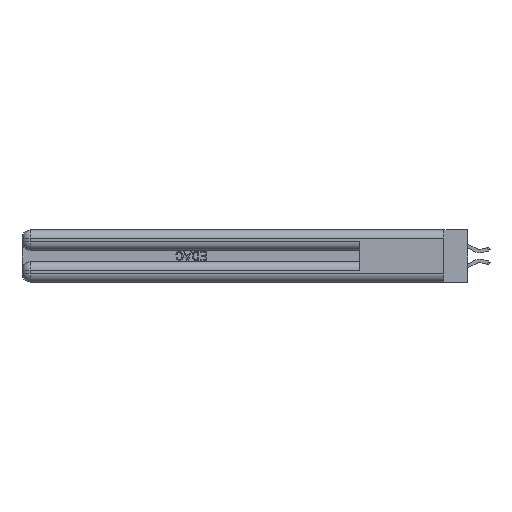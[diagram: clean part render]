
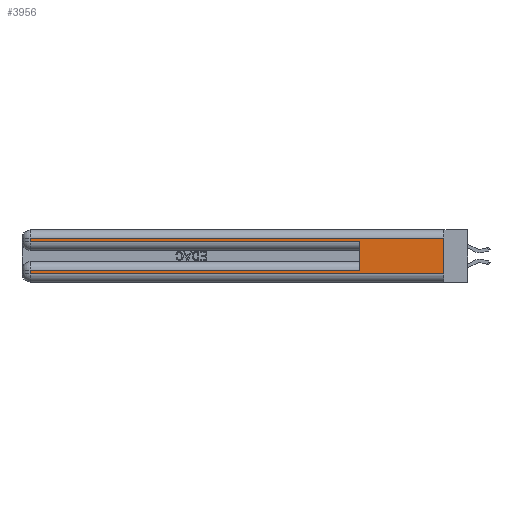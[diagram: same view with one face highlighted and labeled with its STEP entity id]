
A CAD part, left-side view. The second image highlights one B-rep face of the part: STEP entity #3956.
In plain terms, the highlighted planar face has unit normal (-1, 0, 0).
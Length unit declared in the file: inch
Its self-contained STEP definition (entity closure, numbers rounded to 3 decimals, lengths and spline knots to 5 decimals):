
#677 = DIRECTION ( 'NONE',  ( 0., 0., -1. ) ) ;
#1362 = ORIENTED_EDGE ( 'NONE', *, *, #16443, .T. ) ;
#1420 = LINE ( 'NONE', #37237, #9143 ) ;
#2358 = VERTEX_POINT ( 'NONE', #41826 ) ;
#2740 = VECTOR ( 'NONE', #677, 39.37008 ) ;
#3454 = CARTESIAN_POINT ( 'NONE',  ( 0., 0.6, 0.085 ) ) ;
#3956 = ADVANCED_FACE ( 'NONE', ( #18546 ), #12737, .F. ) ;
#4014 = CARTESIAN_POINT ( 'NONE',  ( 0., 2.94, 0.285 ) ) ;
#5277 = EDGE_CURVE ( 'NONE', #16732, #7262, #12969, .T. ) ;
#5862 = ORIENTED_EDGE ( 'NONE', *, *, #5277, .T. ) ;
#5980 = EDGE_CURVE ( 'NONE', #40839, #16732, #20058, .T. ) ;
#6211 = ORIENTED_EDGE ( 'NONE', *, *, #12853, .F. ) ;
#6799 = DIRECTION ( 'NONE',  ( 0., 0., 1. ) ) ;
#7092 = CARTESIAN_POINT ( 'NONE',  ( 0., 2.94, 0.37 ) ) ;
#7262 = VERTEX_POINT ( 'NONE', #27095 ) ;
#8301 = DIRECTION ( 'NONE',  ( 0., -1., 0. ) ) ;
#8622 = DIRECTION ( 'NONE',  ( 0., -1., 0. ) ) ;
#9143 = VECTOR ( 'NONE', #20192, 39.37008 ) ;
#9581 = LINE ( 'NONE', #7092, #37183 ) ;
#10175 = DIRECTION ( 'NONE',  ( 1., 0., 0. ) ) ;
#11609 = EDGE_CURVE ( 'NONE', #2358, #24197, #9581, .T. ) ;
#12737 = PLANE ( 'NONE',  #31847 ) ;
#12807 = ORIENTED_EDGE ( 'NONE', *, *, #5980, .T. ) ;
#12853 = EDGE_CURVE ( 'NONE', #19474, #7262, #25748, .T. ) ;
#12969 = LINE ( 'NONE', #24719, #32415 ) ;
#13239 = CARTESIAN_POINT ( 'NONE',  ( 0., 0., 0.37 ) ) ;
#13685 = CARTESIAN_POINT ( 'NONE',  ( 0., 2.94, 0.37 ) ) ;
#15417 = CARTESIAN_POINT ( 'NONE',  ( 0., 0., 0.37 ) ) ;
#15779 = ORIENTED_EDGE ( 'NONE', *, *, #11609, .T. ) ;
#16417 = CARTESIAN_POINT ( 'NONE',  ( 0., 0.6, 0.145 ) ) ;
#16443 = EDGE_CURVE ( 'NONE', #19474, #2358, #1420, .T. ) ;
#16732 = VERTEX_POINT ( 'NONE', #38180 ) ;
#18546 = FACE_OUTER_BOUND ( 'NONE', #22154, .T. ) ;
#19016 = ORIENTED_EDGE ( 'NONE', *, *, #34197, .T. ) ;
#19474 = VERTEX_POINT ( 'NONE', #27187 ) ;
#20058 = LINE ( 'NONE', #13685, #2740 ) ;
#20192 = DIRECTION ( 'NONE',  ( 0., 1., 0. ) ) ;
#20369 = CARTESIAN_POINT ( 'NONE',  ( 0., 0., 0.285 ) ) ;
#21607 = CARTESIAN_POINT ( 'NONE',  ( 0., 0., 0.085 ) ) ;
#22091 = LINE ( 'NONE', #16417, #39507 ) ;
#22154 = EDGE_LOOP ( 'NONE', ( #6211, #1362, #15779, #26830, #25198, #19016, #12807, #5862 ) ) ;
#23010 = DIRECTION ( 'NONE',  ( 0., 0., -1. ) ) ;
#24197 = VERTEX_POINT ( 'NONE', #4014 ) ;
#24719 = CARTESIAN_POINT ( 'NONE',  ( 0., 0., 0.06 ) ) ;
#24975 = LINE ( 'NONE', #21607, #38297 ) ;
#25198 = ORIENTED_EDGE ( 'NONE', *, *, #36898, .F. ) ;
#25748 = LINE ( 'NONE', #13239, #38604 ) ;
#26830 = ORIENTED_EDGE ( 'NONE', *, *, #33508, .T. ) ;
#27095 = CARTESIAN_POINT ( 'NONE',  ( 0., 0., 0.06 ) ) ;
#27187 = CARTESIAN_POINT ( 'NONE',  ( 0., 0., 0.31 ) ) ;
#28075 = LINE ( 'NONE', #20369, #29642 ) ;
#29307 = CARTESIAN_POINT ( 'NONE',  ( 0., 0.6, 0.285 ) ) ;
#29642 = VECTOR ( 'NONE', #8301, 39.37008 ) ;
#30228 = VERTEX_POINT ( 'NONE', #29307 ) ;
#31847 = AXIS2_PLACEMENT_3D ( 'NONE', #15417, #10175, #23010 ) ;
#32262 = CARTESIAN_POINT ( 'NONE',  ( 0., 2.94, 0.085 ) ) ;
#32415 = VECTOR ( 'NONE', #8622, 39.37008 ) ;
#32531 = DIRECTION ( 'NONE',  ( 0., 0., -1. ) ) ;
#33508 = EDGE_CURVE ( 'NONE', #24197, #30228, #28075, .T. ) ;
#34197 = EDGE_CURVE ( 'NONE', #39916, #40839, #24975, .T. ) ;
#36898 = EDGE_CURVE ( 'NONE', #39916, #30228, #22091, .T. ) ;
#37183 = VECTOR ( 'NONE', #39652, 39.37008 ) ;
#37237 = CARTESIAN_POINT ( 'NONE',  ( 0., 0., 0.31 ) ) ;
#38180 = CARTESIAN_POINT ( 'NONE',  ( 0., 2.94, 0.06 ) ) ;
#38297 = VECTOR ( 'NONE', #41562, 39.37008 ) ;
#38604 = VECTOR ( 'NONE', #32531, 39.37008 ) ;
#39507 = VECTOR ( 'NONE', #6799, 39.37008 ) ;
#39652 = DIRECTION ( 'NONE',  ( 0., 0., -1. ) ) ;
#39916 = VERTEX_POINT ( 'NONE', #3454 ) ;
#40839 = VERTEX_POINT ( 'NONE', #32262 ) ;
#41562 = DIRECTION ( 'NONE',  ( 0., 1., 0. ) ) ;
#41826 = CARTESIAN_POINT ( 'NONE',  ( 0., 2.94, 0.31 ) ) ;
